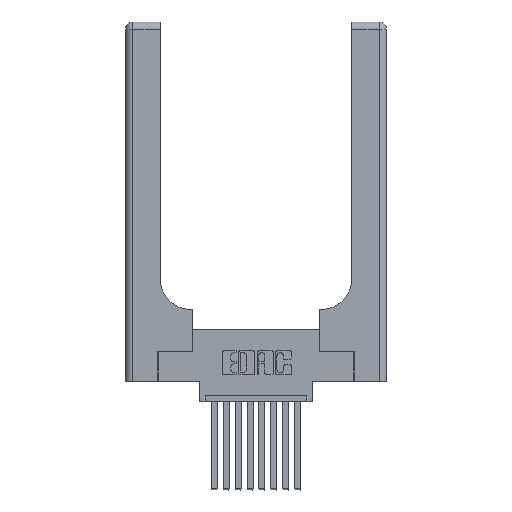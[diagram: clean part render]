
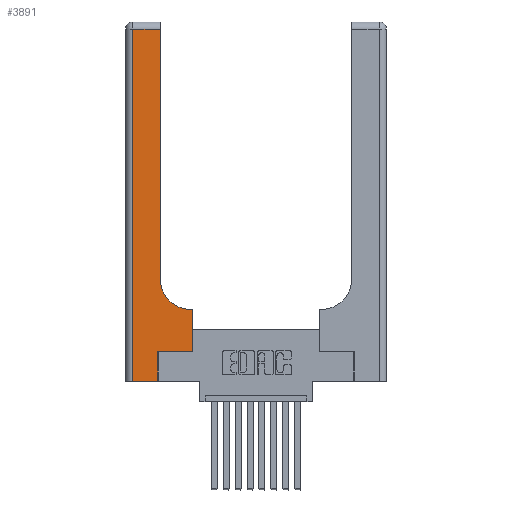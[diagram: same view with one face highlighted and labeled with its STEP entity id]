
A CAD part, top view. The second image highlights one B-rep face of the part: STEP entity #3891.
In plain terms, the highlighted planar face has unit normal (0, 0, 1).
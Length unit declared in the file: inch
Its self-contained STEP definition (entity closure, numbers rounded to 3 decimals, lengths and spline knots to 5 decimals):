
#65 = VERTEX_POINT ( 'NONE', #1106 ) ;
#174 = DIRECTION ( 'NONE',  ( 1., 0., 0. ) ) ;
#225 = LINE ( 'NONE', #8686, #15039 ) ;
#232 = VECTOR ( 'NONE', #12551, 39.37008 ) ;
#261 = EDGE_CURVE ( 'NONE', #13516, #2689, #11609, .T. ) ;
#428 = PLANE ( 'NONE',  #14806 ) ;
#560 = DIRECTION ( 'NONE',  ( 1., 0., 0. ) ) ;
#565 = EDGE_CURVE ( 'NONE', #2689, #10288, #3417, .T. ) ;
#627 = CARTESIAN_POINT ( 'NONE',  ( 0.5585, 0.25, 0.37 ) ) ;
#644 = ORIENTED_EDGE ( 'NONE', *, *, #13234, .T. ) ;
#781 = ORIENTED_EDGE ( 'NONE', *, *, #5909, .T. ) ;
#858 = CARTESIAN_POINT ( 'NONE',  ( 0.2915, 0.6, 0.37 ) ) ;
#1106 = CARTESIAN_POINT ( 'NONE',  ( 0.269, 0.25, 0.37 ) ) ;
#1117 = AXIS2_PLACEMENT_3D ( 'NONE', #12788, #6742, #560 ) ;
#1432 = DIRECTION ( 'NONE',  ( 1., 0., 0. ) ) ;
#1695 = EDGE_CURVE ( 'NONE', #9283, #4116, #11663, .T. ) ;
#1867 = CARTESIAN_POINT ( 'NONE',  ( 0.269, 0., 0.37 ) ) ;
#2007 = ORIENTED_EDGE ( 'NONE', *, *, #565, .T. ) ;
#2454 = CARTESIAN_POINT ( 'NONE',  ( 0.06, 3., 0.37 ) ) ;
#2572 = EDGE_LOOP ( 'NONE', ( #14685, #2007, #11827, #11761, #644, #4929, #781, #3429, #13299 ) ) ;
#2689 = VERTEX_POINT ( 'NONE', #4856 ) ;
#3417 = LINE ( 'NONE', #4075, #232 ) ;
#3429 = ORIENTED_EDGE ( 'NONE', *, *, #10777, .T. ) ;
#3607 = VECTOR ( 'NONE', #6114, 39.37008 ) ;
#3813 = EDGE_CURVE ( 'NONE', #65, #4809, #7587, .T. ) ;
#3891 = ADVANCED_FACE ( 'NONE', ( #15230 ), #428, .F. ) ;
#4075 = CARTESIAN_POINT ( 'NONE',  ( 0., 2.94, 0.37 ) ) ;
#4116 = VERTEX_POINT ( 'NONE', #1867 ) ;
#4218 = VECTOR ( 'NONE', #10895, 39.37008 ) ;
#4564 = CARTESIAN_POINT ( 'NONE',  ( 0.2915, 0.85, 0.37 ) ) ;
#4809 = VERTEX_POINT ( 'NONE', #627 ) ;
#4856 = CARTESIAN_POINT ( 'NONE',  ( 0.2915, 2.94, 0.37 ) ) ;
#4929 = ORIENTED_EDGE ( 'NONE', *, *, #3813, .T. ) ;
#5043 = CARTESIAN_POINT ( 'NONE',  ( 0.06, 0., 0.37 ) ) ;
#5068 = CARTESIAN_POINT ( 'NONE',  ( 0., 3., 0.37 ) ) ;
#5172 = DIRECTION ( 'NONE',  ( -1., 0., 0. ) ) ;
#5556 = CIRCLE ( 'NONE', #1117, 0.25 ) ;
#5559 = LINE ( 'NONE', #2454, #4218 ) ;
#5777 = CARTESIAN_POINT ( 'NONE',  ( 0.5415, 0.6, 0.37 ) ) ;
#5909 = EDGE_CURVE ( 'NONE', #4809, #13448, #10740, .T. ) ;
#5921 = VECTOR ( 'NONE', #8128, 39.37008 ) ;
#6114 = DIRECTION ( 'NONE',  ( 0., 1., 0. ) ) ;
#6199 = CARTESIAN_POINT ( 'NONE',  ( 0.269, 0.25, 0.37 ) ) ;
#6742 = DIRECTION ( 'NONE',  ( 0., 0., -1. ) ) ;
#7541 = VECTOR ( 'NONE', #10515, 39.37008 ) ;
#7587 = LINE ( 'NONE', #6199, #8900 ) ;
#8128 = DIRECTION ( 'NONE',  ( -1., 0., 0. ) ) ;
#8418 = VECTOR ( 'NONE', #1432, 39.37008 ) ;
#8545 = CARTESIAN_POINT ( 'NONE',  ( 0.2915, 3., 0.37 ) ) ;
#8686 = CARTESIAN_POINT ( 'NONE',  ( 0.269, 0., 0.37 ) ) ;
#8776 = DIRECTION ( 'NONE',  ( 0., 0., -1. ) ) ;
#8900 = VECTOR ( 'NONE', #174, 39.37008 ) ;
#9283 = VERTEX_POINT ( 'NONE', #5043 ) ;
#10288 = VERTEX_POINT ( 'NONE', #10774 ) ;
#10515 = DIRECTION ( 'NONE',  ( 0., 1., 0. ) ) ;
#10740 = LINE ( 'NONE', #12693, #7541 ) ;
#10774 = CARTESIAN_POINT ( 'NONE',  ( 0.06, 2.94, 0.37 ) ) ;
#10777 = EDGE_CURVE ( 'NONE', #13448, #14837, #11807, .T. ) ;
#10895 = DIRECTION ( 'NONE',  ( 0., -1., 0. ) ) ;
#11609 = LINE ( 'NONE', #8545, #3607 ) ;
#11663 = LINE ( 'NONE', #12292, #8418 ) ;
#11761 = ORIENTED_EDGE ( 'NONE', *, *, #1695, .T. ) ;
#11807 = LINE ( 'NONE', #858, #5921 ) ;
#11827 = ORIENTED_EDGE ( 'NONE', *, *, #15754, .T. ) ;
#12292 = CARTESIAN_POINT ( 'NONE',  ( 0., 0., 0.37 ) ) ;
#12551 = DIRECTION ( 'NONE',  ( -1., 0., 0. ) ) ;
#12693 = CARTESIAN_POINT ( 'NONE',  ( 0.5585, 0.25, 0.37 ) ) ;
#12788 = CARTESIAN_POINT ( 'NONE',  ( 0.5415, 0.85, 0.37 ) ) ;
#13234 = EDGE_CURVE ( 'NONE', #4116, #65, #225, .T. ) ;
#13299 = ORIENTED_EDGE ( 'NONE', *, *, #15196, .T. ) ;
#13448 = VERTEX_POINT ( 'NONE', #14254 ) ;
#13516 = VERTEX_POINT ( 'NONE', #4564 ) ;
#13602 = DIRECTION ( 'NONE',  ( 0., 1., 0. ) ) ;
#14254 = CARTESIAN_POINT ( 'NONE',  ( 0.5585, 0.6, 0.37 ) ) ;
#14685 = ORIENTED_EDGE ( 'NONE', *, *, #261, .T. ) ;
#14806 = AXIS2_PLACEMENT_3D ( 'NONE', #5068, #8776, #5172 ) ;
#14837 = VERTEX_POINT ( 'NONE', #5777 ) ;
#15039 = VECTOR ( 'NONE', #13602, 39.37008 ) ;
#15196 = EDGE_CURVE ( 'NONE', #14837, #13516, #5556, .T. ) ;
#15230 = FACE_OUTER_BOUND ( 'NONE', #2572, .T. ) ;
#15754 = EDGE_CURVE ( 'NONE', #10288, #9283, #5559, .T. ) ;
